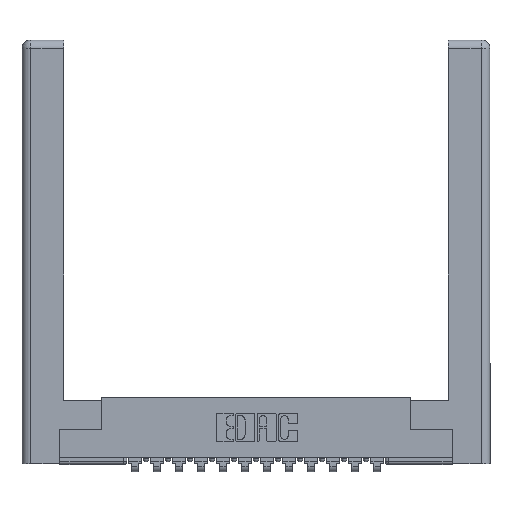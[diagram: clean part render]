
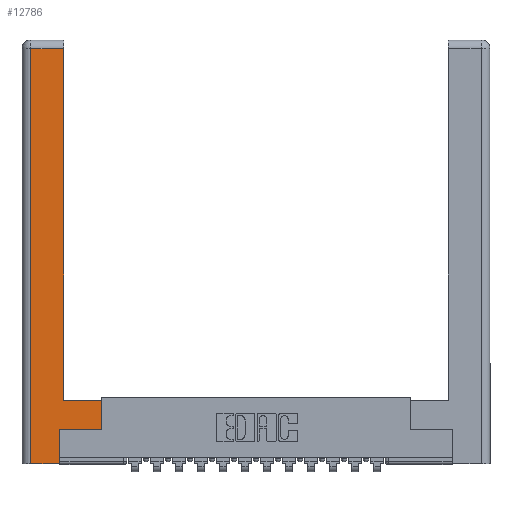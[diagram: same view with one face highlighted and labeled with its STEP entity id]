
A CAD part, top view. The second image highlights one B-rep face of the part: STEP entity #12786.
In plain terms, the highlighted planar face has unit normal (0, 0, 1).
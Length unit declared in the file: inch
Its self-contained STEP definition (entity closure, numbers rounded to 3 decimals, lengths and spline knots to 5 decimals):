
#45 = EDGE_CURVE ( 'NONE', #568, #4363, #8881, .T. ) ;
#219 = VECTOR ( 'NONE', #2767, 39.37008 ) ;
#273 = LINE ( 'NONE', #17414, #15239 ) ;
#420 = DIRECTION ( 'NONE',  ( -1., 0., 0. ) ) ;
#568 = VERTEX_POINT ( 'NONE', #16351 ) ;
#1038 = VERTEX_POINT ( 'NONE', #3142 ) ;
#1485 = CARTESIAN_POINT ( 'NONE',  ( 0.265, 0.245, 0. ) ) ;
#1511 = EDGE_CURVE ( 'NONE', #15329, #1038, #11793, .T. ) ;
#1716 = VERTEX_POINT ( 'NONE', #10100 ) ;
#1813 = ORIENTED_EDGE ( 'NONE', *, *, #1511, .T. ) ;
#1822 = DIRECTION ( 'NONE',  ( 1., 0., 0. ) ) ;
#1992 = EDGE_CURVE ( 'NONE', #14881, #1716, #16835, .T. ) ;
#2093 = LINE ( 'NONE', #1485, #7354 ) ;
#2165 = VECTOR ( 'NONE', #1822, 39.37008 ) ;
#2300 = CARTESIAN_POINT ( 'NONE',  ( 0., 0., 0. ) ) ;
#2767 = DIRECTION ( 'NONE',  ( 0., 1., 0. ) ) ;
#2775 = CARTESIAN_POINT ( 'NONE',  ( 0.265, 0.245, 0. ) ) ;
#3142 = CARTESIAN_POINT ( 'NONE',  ( 0.565, 0.245, 0. ) ) ;
#3343 = EDGE_CURVE ( 'NONE', #1716, #568, #8315, .T. ) ;
#3594 = VECTOR ( 'NONE', #12405, 39.37008 ) ;
#3677 = ORIENTED_EDGE ( 'NONE', *, *, #7390, .T. ) ;
#3790 = ORIENTED_EDGE ( 'NONE', *, *, #3343, .T. ) ;
#4363 = VERTEX_POINT ( 'NONE', #10804 ) ;
#4407 = EDGE_LOOP ( 'NONE', ( #16530, #12082, #3790, #10568, #3677, #1813, #14136, #16743 ) ) ;
#4608 = DIRECTION ( 'NONE',  ( -1., 0., 0. ) ) ;
#4861 = LINE ( 'NONE', #8154, #219 ) ;
#4948 = EDGE_CURVE ( 'NONE', #13081, #14881, #273, .T. ) ;
#6124 = AXIS2_PLACEMENT_3D ( 'NONE', #2300, #6361, #7751 ) ;
#6361 = DIRECTION ( 'NONE',  ( 0., 0., -1. ) ) ;
#7354 = VECTOR ( 'NONE', #9408, 39.37008 ) ;
#7390 = EDGE_CURVE ( 'NONE', #4363, #15329, #2093, .T. ) ;
#7638 = VERTEX_POINT ( 'NONE', #8639 ) ;
#7751 = DIRECTION ( 'NONE',  ( -1., 0., 0. ) ) ;
#8151 = CARTESIAN_POINT ( 'NONE',  ( 0.295, 0.45, 0. ) ) ;
#8154 = CARTESIAN_POINT ( 'NONE',  ( 0.565, 0.45, 0. ) ) ;
#8315 = LINE ( 'NONE', #16286, #13374 ) ;
#8334 = EDGE_CURVE ( 'NONE', #1038, #7638, #4861, .T. ) ;
#8571 = CARTESIAN_POINT ( 'NONE',  ( 0.295, 0.45, 0. ) ) ;
#8639 = CARTESIAN_POINT ( 'NONE',  ( 0.565, 0.45, 0. ) ) ;
#8685 = CARTESIAN_POINT ( 'NONE',  ( 0.265, 0., 0. ) ) ;
#8721 = CARTESIAN_POINT ( 'NONE',  ( 0.295, 2.94, 0. ) ) ;
#8755 = EDGE_CURVE ( 'NONE', #7638, #13081, #17078, .T. ) ;
#8881 = LINE ( 'NONE', #8685, #2165 ) ;
#9408 = DIRECTION ( 'NONE',  ( 0., 1., 0. ) ) ;
#10100 = CARTESIAN_POINT ( 'NONE',  ( 0.0615, 2.94, 0. ) ) ;
#10568 = ORIENTED_EDGE ( 'NONE', *, *, #45, .T. ) ;
#10804 = CARTESIAN_POINT ( 'NONE',  ( 0.265, 0., 0. ) ) ;
#11060 = CARTESIAN_POINT ( 'NONE',  ( 0.0615, 2.94, 0. ) ) ;
#11764 = PLANE ( 'NONE',  #6124 ) ;
#11793 = LINE ( 'NONE', #13640, #3594 ) ;
#12082 = ORIENTED_EDGE ( 'NONE', *, *, #1992, .T. ) ;
#12405 = DIRECTION ( 'NONE',  ( 1., 0., 0. ) ) ;
#12786 = ADVANCED_FACE ( 'NONE', ( #16325 ), #11764, .F. ) ;
#13081 = VERTEX_POINT ( 'NONE', #8151 ) ;
#13374 = VECTOR ( 'NONE', #13604, 39.37008 ) ;
#13454 = VECTOR ( 'NONE', #4608, 39.37008 ) ;
#13604 = DIRECTION ( 'NONE',  ( 0., -1., 0. ) ) ;
#13640 = CARTESIAN_POINT ( 'NONE',  ( 0.565, 0.245, 0. ) ) ;
#14136 = ORIENTED_EDGE ( 'NONE', *, *, #8334, .T. ) ;
#14881 = VERTEX_POINT ( 'NONE', #8721 ) ;
#15239 = VECTOR ( 'NONE', #17468, 39.37008 ) ;
#15329 = VERTEX_POINT ( 'NONE', #2775 ) ;
#16218 = VECTOR ( 'NONE', #420, 39.37008 ) ;
#16286 = CARTESIAN_POINT ( 'NONE',  ( 0.0615, 0., 0. ) ) ;
#16325 = FACE_OUTER_BOUND ( 'NONE', #4407, .T. ) ;
#16351 = CARTESIAN_POINT ( 'NONE',  ( 0.0615, 0., 0. ) ) ;
#16530 = ORIENTED_EDGE ( 'NONE', *, *, #4948, .T. ) ;
#16743 = ORIENTED_EDGE ( 'NONE', *, *, #8755, .T. ) ;
#16835 = LINE ( 'NONE', #11060, #16218 ) ;
#17078 = LINE ( 'NONE', #8571, #13454 ) ;
#17414 = CARTESIAN_POINT ( 'NONE',  ( 0.295, 3., 0. ) ) ;
#17468 = DIRECTION ( 'NONE',  ( 0., 1., 0. ) ) ;
